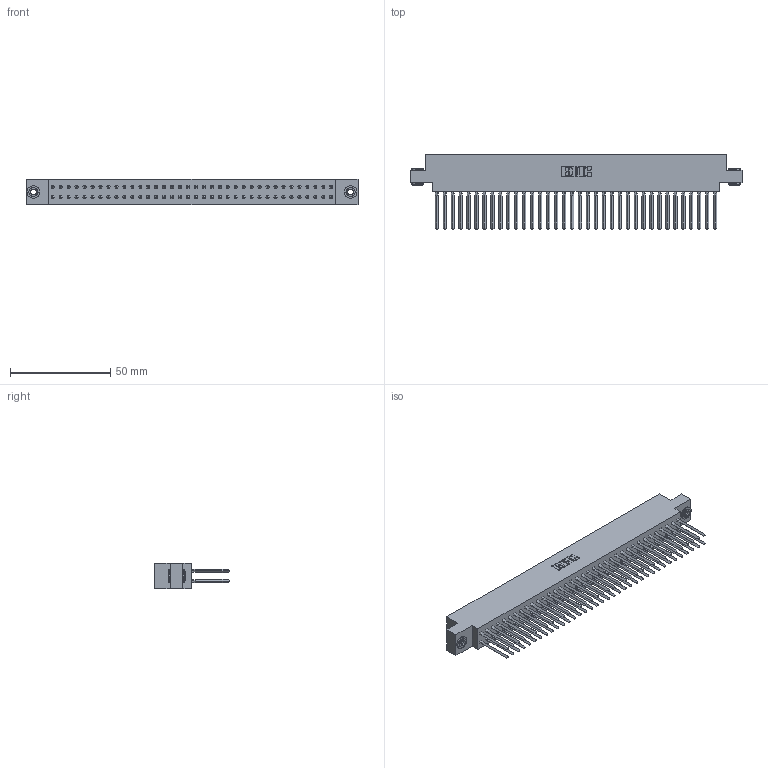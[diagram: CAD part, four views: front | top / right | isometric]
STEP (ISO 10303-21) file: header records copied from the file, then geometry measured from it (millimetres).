
FILE_DESCRIPTION (( 'STEP AP203' ), '1' );
FILE_NAME ('317-072-540-803.STEP', '2020-02-28T07:23:30', ( '' ), ( '' ), 'SwSTEP 2.0', 'SolidWorks 2016', '' );
FILE_SCHEMA (( 'CONFIG_CONTROL_DESIGN' ));
Length unit declared in the file: inch
Products named in the file (4): 345-250-002_345-250-002-102; 317 Part_.156 Dia - TH; 317-072-540-803; 317-290-001_540
Assembly tree (75 placements, depth 2):
  317-072-540-803
    317 Part_.156 Dia - TH
    317-290-001_540  x72
    345-250-002_345-250-002-102  x2
Bounding box: 165.35 x 37.34 x 12.7 mm (x, y, z)
Volume: 27568.1 mm3; surface area: 41088.3 mm2
Topology: 75 solids, 75 shells, 6548 faces, 18135 edges, 11678 vertices
Faces by surface type: plane 5324, cylinder 928, bspline 288, cone 8
Entity records: 53525 total; most frequent: CARTESIAN_POINT 9722, ORIENTED_EDGE 9214, DIRECTION 7727, EDGE_CURVE 4607, VECTOR 4327, LINE 4327, VERTEX_POINT 3063, AXIS2_PLACEMENT_3D 1700
